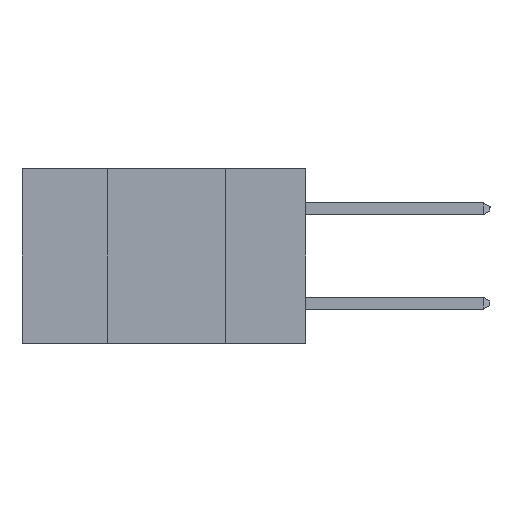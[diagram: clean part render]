
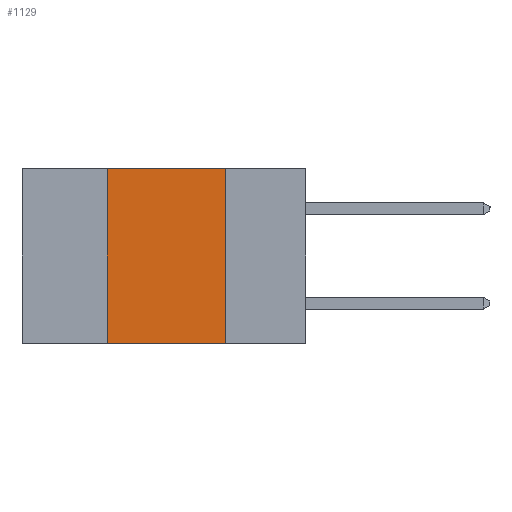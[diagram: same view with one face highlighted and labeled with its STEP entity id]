
A CAD part, left-side view. The second image highlights one B-rep face of the part: STEP entity #1129.
In plain terms, the highlighted planar face has unit normal (-1, 0, 0).
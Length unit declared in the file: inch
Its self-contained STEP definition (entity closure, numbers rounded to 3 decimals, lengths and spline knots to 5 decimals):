
#43 = CARTESIAN_POINT ( 'NONE',  ( 0., 0.17, -0.37 ) ) ;
#496 = EDGE_CURVE ( 'NONE', #3763, #17302, #20066, .T. ) ;
#673 = CARTESIAN_POINT ( 'NONE',  ( 0., 0.42, -0.37 ) ) ;
#1106 = ORIENTED_EDGE ( 'NONE', *, *, #7538, .T. ) ;
#1114 = VERTEX_POINT ( 'NONE', #43 ) ;
#1129 = ADVANCED_FACE ( 'NONE', ( #11239 ), #17632, .F. ) ;
#1852 = VECTOR ( 'NONE', #3624, 39.37008 ) ;
#2105 = EDGE_CURVE ( 'NONE', #17302, #1114, #9994, .T. ) ;
#3435 = EDGE_LOOP ( 'NONE', ( #6107, #4099, #7239, #1106 ) ) ;
#3595 = CARTESIAN_POINT ( 'NONE',  ( 0., 0.17, 0. ) ) ;
#3624 = DIRECTION ( 'NONE',  ( 0., 0., -1. ) ) ;
#3763 = VERTEX_POINT ( 'NONE', #14299 ) ;
#3886 = AXIS2_PLACEMENT_3D ( 'NONE', #16064, #10921, #8103 ) ;
#4099 = ORIENTED_EDGE ( 'NONE', *, *, #496, .F. ) ;
#4199 = VERTEX_POINT ( 'NONE', #673 ) ;
#5170 = EDGE_CURVE ( 'NONE', #4199, #3763, #8839, .T. ) ;
#5698 = DIRECTION ( 'NONE',  ( 0., 0., 1. ) ) ;
#6107 = ORIENTED_EDGE ( 'NONE', *, *, #2105, .F. ) ;
#7239 = ORIENTED_EDGE ( 'NONE', *, *, #5170, .F. ) ;
#7538 = EDGE_CURVE ( 'NONE', #4199, #1114, #12343, .T. ) ;
#7601 = DIRECTION ( 'NONE',  ( 0., -1., 0. ) ) ;
#7802 = VECTOR ( 'NONE', #7601, 39.37008 ) ;
#8103 = DIRECTION ( 'NONE',  ( 0., 0., -1. ) ) ;
#8839 = LINE ( 'NONE', #9041, #15698 ) ;
#9041 = CARTESIAN_POINT ( 'NONE',  ( 0., 0.42, -0.37 ) ) ;
#9994 = LINE ( 'NONE', #13240, #1852 ) ;
#10452 = DIRECTION ( 'NONE',  ( 0., -1., 0. ) ) ;
#10921 = DIRECTION ( 'NONE',  ( 1., 0., 0. ) ) ;
#11239 = FACE_OUTER_BOUND ( 'NONE', #3435, .T. ) ;
#12116 = CARTESIAN_POINT ( 'NONE',  ( 0., 0.6, 0. ) ) ;
#12343 = LINE ( 'NONE', #19989, #14613 ) ;
#13240 = CARTESIAN_POINT ( 'NONE',  ( 0., 0.17, -0.37 ) ) ;
#14299 = CARTESIAN_POINT ( 'NONE',  ( 0., 0.42, 0. ) ) ;
#14613 = VECTOR ( 'NONE', #10452, 39.37008 ) ;
#15698 = VECTOR ( 'NONE', #5698, 39.37008 ) ;
#16064 = CARTESIAN_POINT ( 'NONE',  ( 0., 0.6, 0. ) ) ;
#17302 = VERTEX_POINT ( 'NONE', #3595 ) ;
#17632 = PLANE ( 'NONE',  #3886 ) ;
#19989 = CARTESIAN_POINT ( 'NONE',  ( 0., 0.6, -0.37 ) ) ;
#20066 = LINE ( 'NONE', #12116, #7802 ) ;
